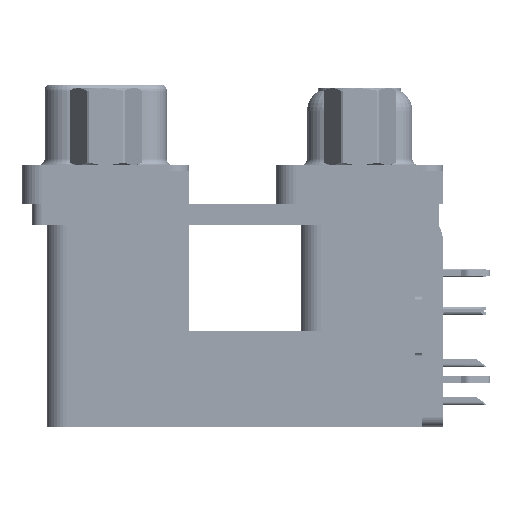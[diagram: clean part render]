
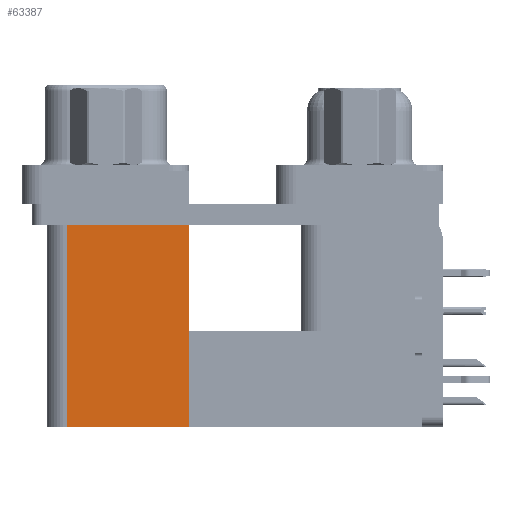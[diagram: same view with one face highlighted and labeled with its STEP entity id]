
A CAD part, left-side view. The second image highlights one B-rep face of the part: STEP entity #63387.
In plain terms, the highlighted planar face has unit normal (-1, 0, 0).
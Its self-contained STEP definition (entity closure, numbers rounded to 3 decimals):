
#1284 = AXIS2_PLACEMENT_3D ( 'NONE', #46484, #74224, #27874 ) ;
#8350 = CARTESIAN_POINT ( 'NONE',  ( 3.79, 12.775, -19.2 ) ) ;
#8702 = VERTEX_POINT ( 'NONE', #8350 ) ;
#11101 = FACE_OUTER_BOUND ( 'NONE', #67730, .T. ) ;
#16239 = LINE ( 'NONE', #62633, #74875 ) ;
#20260 = DIRECTION ( 'NONE',  ( 0., 0., 1. ) ) ;
#21417 = ORIENTED_EDGE ( 'NONE', *, *, #56390, .T. ) ;
#21906 = VECTOR ( 'NONE', #20260, 1000. ) ;
#22556 = VERTEX_POINT ( 'NONE', #29350 ) ;
#23161 = CARTESIAN_POINT ( 'NONE',  ( 3.79, 12.775, -2.5 ) ) ;
#27874 = DIRECTION ( 'NONE',  ( 0., 1., 0. ) ) ;
#29070 = VECTOR ( 'NONE', #38231, 1000. ) ;
#29350 = CARTESIAN_POINT ( 'NONE',  ( 3.79, 21.975, -2.5 ) ) ;
#30862 = VECTOR ( 'NONE', #65563, 1000. ) ;
#38231 = DIRECTION ( 'NONE',  ( 0., 1., 0. ) ) ;
#39227 = VERTEX_POINT ( 'NONE', #23161 ) ;
#40927 = LINE ( 'NONE', #71258, #30862 ) ;
#45296 = EDGE_CURVE ( 'NONE', #73312, #22556, #40927, .T. ) ;
#46484 = CARTESIAN_POINT ( 'NONE',  ( 3.79, 12.775, -19.2 ) ) ;
#49032 = ORIENTED_EDGE ( 'NONE', *, *, #54869, .F. ) ;
#49165 = CARTESIAN_POINT ( 'NONE',  ( 3.79, 12.775, -19.2 ) ) ;
#52619 = ORIENTED_EDGE ( 'NONE', *, *, #45296, .F. ) ;
#54869 = EDGE_CURVE ( 'NONE', #8702, #73312, #61411, .T. ) ;
#55625 = LINE ( 'NONE', #49165, #21906 ) ;
#56390 = EDGE_CURVE ( 'NONE', #39227, #22556, #16239, .T. ) ;
#60217 = ORIENTED_EDGE ( 'NONE', *, *, #64666, .T. ) ;
#61411 = LINE ( 'NONE', #71765, #29070 ) ;
#62633 = CARTESIAN_POINT ( 'NONE',  ( 3.79, 12.775, -2.5 ) ) ;
#63213 = PLANE ( 'NONE',  #1284 ) ;
#63387 = ADVANCED_FACE ( 'NONE', ( #11101 ), #63213, .F. ) ;
#64666 = EDGE_CURVE ( 'NONE', #8702, #39227, #55625, .T. ) ;
#65563 = DIRECTION ( 'NONE',  ( 0., 0., 1. ) ) ;
#67730 = EDGE_LOOP ( 'NONE', ( #21417, #52619, #49032, #60217 ) ) ;
#68971 = CARTESIAN_POINT ( 'NONE',  ( 3.79, 21.975, -19.2 ) ) ;
#71258 = CARTESIAN_POINT ( 'NONE',  ( 3.79, 21.975, -19.2 ) ) ;
#71765 = CARTESIAN_POINT ( 'NONE',  ( 3.79, 12.775, -19.2 ) ) ;
#73147 = DIRECTION ( 'NONE',  ( 0., 1., 0. ) ) ;
#73312 = VERTEX_POINT ( 'NONE', #68971 ) ;
#74224 = DIRECTION ( 'NONE',  ( 1., 0., 0. ) ) ;
#74875 = VECTOR ( 'NONE', #73147, 1000. ) ;
